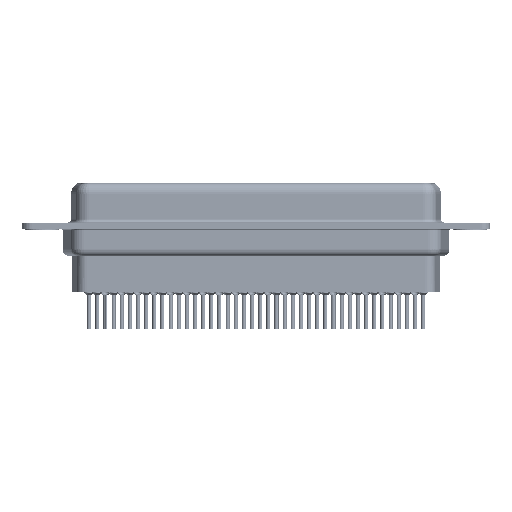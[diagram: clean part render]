
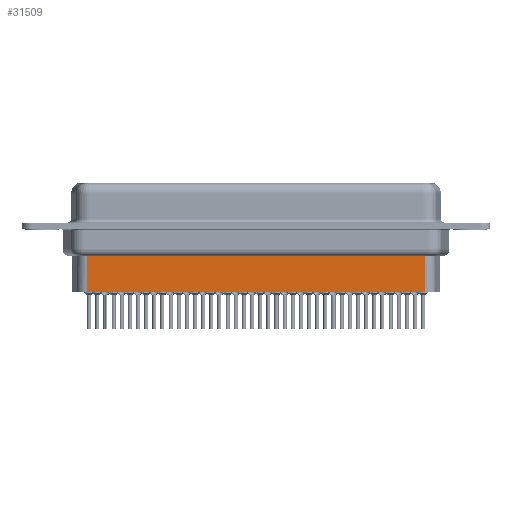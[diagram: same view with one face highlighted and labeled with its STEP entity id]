
A CAD part, front view. The second image highlights one B-rep face of the part: STEP entity #31509.
In plain terms, the highlighted planar face has unit normal (0, -1, 0).
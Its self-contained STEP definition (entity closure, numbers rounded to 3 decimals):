
#3 = CARTESIAN_POINT ( 'NONE',  ( 56.794, -3.5, -4.097 ) ) ;
#714 = CARTESIAN_POINT ( 'NONE',  ( 56.794, -3.5, -3.1 ) ) ;
#1400 = DIRECTION ( 'NONE',  ( 0., 0., -1. ) ) ;
#1657 = EDGE_CURVE ( 'NONE', #3421, #42581, #10077, .T. ) ;
#2932 = EDGE_CURVE ( 'NONE', #3421, #17573, #32014, .T. ) ;
#3421 = VERTEX_POINT ( 'NONE', #3 ) ;
#3864 = CARTESIAN_POINT ( 'NONE',  ( 6.459, -3.5, -4.097 ) ) ;
#4438 = EDGE_CURVE ( 'NONE', #42581, #14140, #5522, .T. ) ;
#5522 = LINE ( 'NONE', #32928, #23144 ) ;
#5737 = ORIENTED_EDGE ( 'NONE', *, *, #4438, .T. ) ;
#6996 = VECTOR ( 'NONE', #17808, 1000. ) ;
#8412 = CARTESIAN_POINT ( 'NONE',  ( 6.706, -3.5, -4.097 ) ) ;
#10077 = LINE ( 'NONE', #3864, #6996 ) ;
#11243 = DIRECTION ( 'NONE',  ( 0., 0., -1. ) ) ;
#12763 = FACE_OUTER_BOUND ( 'NONE', #24481, .T. ) ;
#14140 = VERTEX_POINT ( 'NONE', #15730 ) ;
#15730 = CARTESIAN_POINT ( 'NONE',  ( 6.706, -3.5, -9.85 ) ) ;
#17010 = ORIENTED_EDGE ( 'NONE', *, *, #2932, .F. ) ;
#17132 = LINE ( 'NONE', #41764, #33504 ) ;
#17573 = VERTEX_POINT ( 'NONE', #28182 ) ;
#17808 = DIRECTION ( 'NONE',  ( -1., 0., 0. ) ) ;
#19105 = EDGE_CURVE ( 'NONE', #17573, #14140, #17132, .T. ) ;
#20066 = VECTOR ( 'NONE', #11243, 1000. ) ;
#20974 = DIRECTION ( 'NONE',  ( -1., 0., 0. ) ) ;
#23026 = PLANE ( 'NONE',  #38234 ) ;
#23144 = VECTOR ( 'NONE', #1400, 1000. ) ;
#23246 = DIRECTION ( 'NONE',  ( 1., 0., 0. ) ) ;
#24481 = EDGE_LOOP ( 'NONE', ( #17010, #27020, #5737, #41888 ) ) ;
#26000 = DIRECTION ( 'NONE',  ( 0., -1., 0. ) ) ;
#27020 = ORIENTED_EDGE ( 'NONE', *, *, #1657, .T. ) ;
#28182 = CARTESIAN_POINT ( 'NONE',  ( 56.794, -3.5, -9.85 ) ) ;
#31509 = ADVANCED_FACE ( 'NONE', ( #12763 ), #23026, .T. ) ;
#32014 = LINE ( 'NONE', #714, #20066 ) ;
#32928 = CARTESIAN_POINT ( 'NONE',  ( 6.706, -3.5, -3.1 ) ) ;
#33504 = VECTOR ( 'NONE', #20974, 1000. ) ;
#36950 = CARTESIAN_POINT ( 'NONE',  ( 6.706, -3.5, -3.1 ) ) ;
#38234 = AXIS2_PLACEMENT_3D ( 'NONE', #36950, #26000, #23246 ) ;
#41764 = CARTESIAN_POINT ( 'NONE',  ( 6.706, -3.5, -9.85 ) ) ;
#41888 = ORIENTED_EDGE ( 'NONE', *, *, #19105, .F. ) ;
#42581 = VERTEX_POINT ( 'NONE', #8412 ) ;
